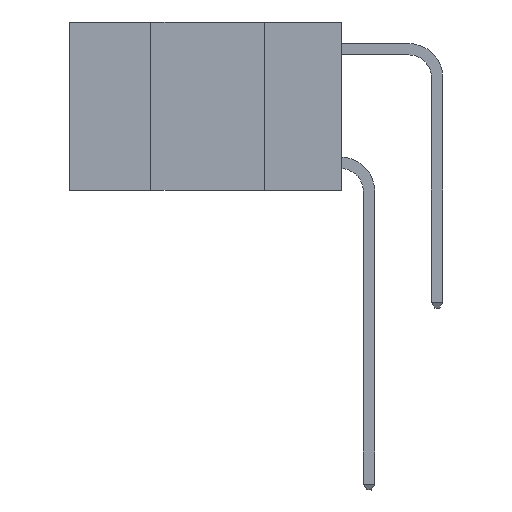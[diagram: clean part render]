
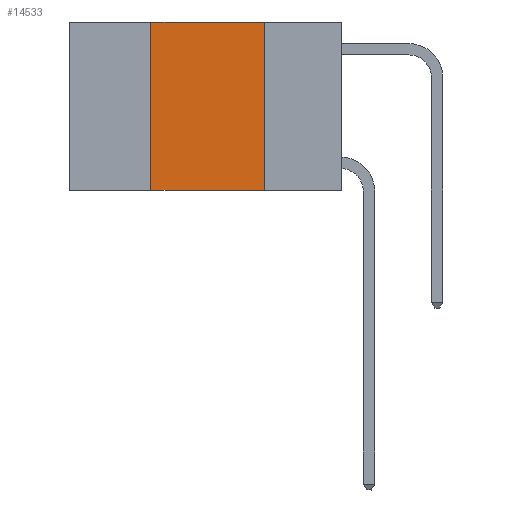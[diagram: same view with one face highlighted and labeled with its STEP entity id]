
A CAD part, left-side view. The second image highlights one B-rep face of the part: STEP entity #14533.
In plain terms, the highlighted planar face has unit normal (-1, 0, 0).
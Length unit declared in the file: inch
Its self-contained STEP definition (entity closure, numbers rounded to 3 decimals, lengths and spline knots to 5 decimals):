
#863 = EDGE_CURVE ( 'NONE', #1871, #999, #8470, .T. ) ;
#999 = VERTEX_POINT ( 'NONE', #9700 ) ;
#1118 = PLANE ( 'NONE',  #9814 ) ;
#1871 = VERTEX_POINT ( 'NONE', #2775 ) ;
#1905 = VERTEX_POINT ( 'NONE', #12562 ) ;
#1989 = DIRECTION ( 'NONE',  ( 0., 0., 1. ) ) ;
#2775 = CARTESIAN_POINT ( 'NONE',  ( 0., 0.42, -0.37 ) ) ;
#3080 = DIRECTION ( 'NONE',  ( 0., 0., -1. ) ) ;
#4147 = EDGE_LOOP ( 'NONE', ( #12006, #10097, #14410, #6535 ) ) ;
#4573 = EDGE_CURVE ( 'NONE', #1871, #1905, #7105, .T. ) ;
#6535 = ORIENTED_EDGE ( 'NONE', *, *, #863, .T. ) ;
#6712 = VECTOR ( 'NONE', #18097, 39.37008 ) ;
#6718 = EDGE_CURVE ( 'NONE', #15653, #999, #12189, .T. ) ;
#6880 = LINE ( 'NONE', #17766, #17604 ) ;
#7105 = LINE ( 'NONE', #14597, #17857 ) ;
#8470 = LINE ( 'NONE', #16726, #6712 ) ;
#9499 = VECTOR ( 'NONE', #3080, 39.37008 ) ;
#9700 = CARTESIAN_POINT ( 'NONE',  ( 0., 0.17, -0.37 ) ) ;
#9814 = AXIS2_PLACEMENT_3D ( 'NONE', #12450, #16951, #11082 ) ;
#10097 = ORIENTED_EDGE ( 'NONE', *, *, #15944, .F. ) ;
#10807 = CARTESIAN_POINT ( 'NONE',  ( 0., 0.17, 0. ) ) ;
#11082 = DIRECTION ( 'NONE',  ( 0., 0., -1. ) ) ;
#12006 = ORIENTED_EDGE ( 'NONE', *, *, #6718, .F. ) ;
#12189 = LINE ( 'NONE', #13191, #9499 ) ;
#12450 = CARTESIAN_POINT ( 'NONE',  ( 0., 0.6, 0. ) ) ;
#12562 = CARTESIAN_POINT ( 'NONE',  ( 0., 0.42, 0. ) ) ;
#13191 = CARTESIAN_POINT ( 'NONE',  ( 0., 0.17, 0. ) ) ;
#14410 = ORIENTED_EDGE ( 'NONE', *, *, #4573, .F. ) ;
#14533 = ADVANCED_FACE ( 'NONE', ( #16298 ), #1118, .F. ) ;
#14597 = CARTESIAN_POINT ( 'NONE',  ( 0., 0.42, 0. ) ) ;
#15653 = VERTEX_POINT ( 'NONE', #10807 ) ;
#15944 = EDGE_CURVE ( 'NONE', #1905, #15653, #6880, .T. ) ;
#16298 = FACE_OUTER_BOUND ( 'NONE', #4147, .T. ) ;
#16726 = CARTESIAN_POINT ( 'NONE',  ( 0., 0.6, -0.37 ) ) ;
#16951 = DIRECTION ( 'NONE',  ( 1., 0., 0. ) ) ;
#17604 = VECTOR ( 'NONE', #18134, 39.37008 ) ;
#17766 = CARTESIAN_POINT ( 'NONE',  ( 0., 0.6, 0. ) ) ;
#17857 = VECTOR ( 'NONE', #1989, 39.37008 ) ;
#18097 = DIRECTION ( 'NONE',  ( 0., -1., 0. ) ) ;
#18134 = DIRECTION ( 'NONE',  ( 0., -1., 0. ) ) ;
